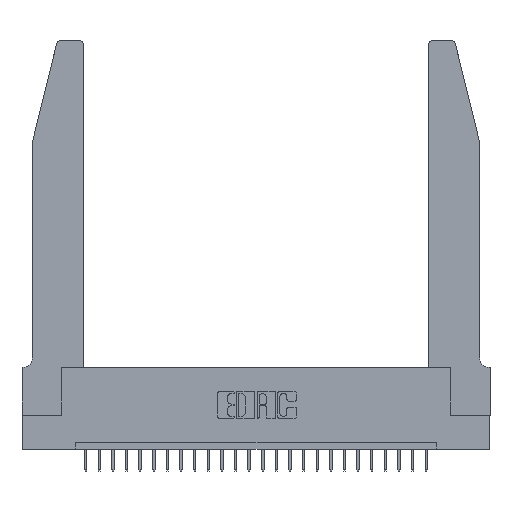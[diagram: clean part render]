
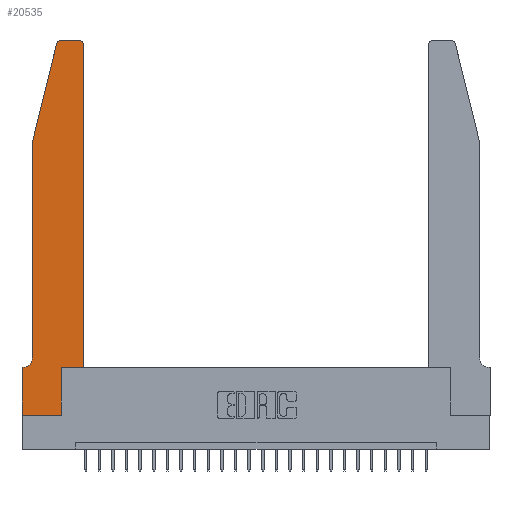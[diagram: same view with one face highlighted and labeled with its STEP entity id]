
A CAD part, top view. The second image highlights one B-rep face of the part: STEP entity #20535.
In plain terms, the highlighted planar face has unit normal (0, 0, 1).
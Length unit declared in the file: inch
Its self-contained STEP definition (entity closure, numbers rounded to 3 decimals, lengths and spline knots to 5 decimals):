
#472 = DIRECTION ( 'NONE',  ( -1., 0., 0. ) ) ;
#567 = CARTESIAN_POINT ( 'NONE',  ( 0.0055, 0.42, 0.37 ) ) ;
#782 = LINE ( 'NONE', #8113, #13665 ) ;
#947 = CARTESIAN_POINT ( 'NONE',  ( 0.25487, 2.72718, 0.37 ) ) ;
#1021 = EDGE_CURVE ( 'NONE', #4574, #17911, #22166, .T. ) ;
#1722 = DIRECTION ( 'NONE',  ( 1., 0., 0. ) ) ;
#2195 = CARTESIAN_POINT ( 'NONE',  ( 0.0055, 0.35, 0.37 ) ) ;
#2310 = AXIS2_PLACEMENT_3D ( 'NONE', #18141, #11943, #11862 ) ;
#2638 = CARTESIAN_POINT ( 'NONE',  ( 0.0755, 0.42, 0.37 ) ) ;
#2735 = DIRECTION ( 'NONE',  ( -1., 0., 0. ) ) ;
#2921 = ORIENTED_EDGE ( 'NONE', *, *, #15101, .T. ) ;
#3608 = ORIENTED_EDGE ( 'NONE', *, *, #18608, .T. ) ;
#3681 = EDGE_CURVE ( 'NONE', #5317, #7916, #22575, .T. ) ;
#3725 = DIRECTION ( 'NONE',  ( 0., 1., 0. ) ) ;
#4243 = AXIS2_PLACEMENT_3D ( 'NONE', #16172, #10070, #22353 ) ;
#4574 = VERTEX_POINT ( 'NONE', #26457 ) ;
#5047 = ORIENTED_EDGE ( 'NONE', *, *, #3681, .T. ) ;
#5179 = VECTOR ( 'NONE', #20657, 39.37008 ) ;
#5317 = VERTEX_POINT ( 'NONE', #20674 ) ;
#5391 = LINE ( 'NONE', #9657, #13701 ) ;
#5473 = DIRECTION ( 'NONE',  ( 1., 0., 0. ) ) ;
#5727 = CARTESIAN_POINT ( 'NONE',  ( 0., 0.35, 0.37 ) ) ;
#5961 = CARTESIAN_POINT ( 'NONE',  ( 0.4505, 0.35, 0.37 ) ) ;
#5993 = ORIENTED_EDGE ( 'NONE', *, *, #10647, .T. ) ;
#6028 = EDGE_LOOP ( 'NONE', ( #17126, #25659, #2921, #17463, #17440, #12930, #3608, #5993, #26164, #24307, #5047, #20089 ) ) ;
#6051 = DIRECTION ( 'NONE',  ( 0., 1., 0. ) ) ;
#6361 = CARTESIAN_POINT ( 'NONE',  ( 0.0755, 2., 0.37 ) ) ;
#6406 = CARTESIAN_POINT ( 'NONE',  ( 0., 0., 0.37 ) ) ;
#6776 = DIRECTION ( 'NONE',  ( 1., 0., 0. ) ) ;
#6785 = VERTEX_POINT ( 'NONE', #19899 ) ;
#7282 = CARTESIAN_POINT ( 'NONE',  ( 0., 0., 0.37 ) ) ;
#7431 = CARTESIAN_POINT ( 'NONE',  ( 0.0755, 2., 0.37 ) ) ;
#7916 = VERTEX_POINT ( 'NONE', #19694 ) ;
#8113 = CARTESIAN_POINT ( 'NONE',  ( 0.2865, 0.35, 0.37 ) ) ;
#8120 = VERTEX_POINT ( 'NONE', #23173 ) ;
#8487 = EDGE_CURVE ( 'NONE', #6785, #10697, #9330, .T. ) ;
#9235 = LINE ( 'NONE', #7431, #21674 ) ;
#9330 = LINE ( 'NONE', #6361, #5179 ) ;
#9657 = CARTESIAN_POINT ( 'NONE',  ( 0.0755, 0.35, 0.37 ) ) ;
#9749 = PLANE ( 'NONE',  #23344 ) ;
#10070 = DIRECTION ( 'NONE',  ( 0., 0., 1. ) ) ;
#10303 = CARTESIAN_POINT ( 'NONE',  ( 0., 0.35, 0.37 ) ) ;
#10463 = FACE_OUTER_BOUND ( 'NONE', #6028, .T. ) ;
#10647 = EDGE_CURVE ( 'NONE', #8120, #23838, #16918, .T. ) ;
#10697 = VERTEX_POINT ( 'NONE', #2638 ) ;
#11446 = VERTEX_POINT ( 'NONE', #10303 ) ;
#11862 = DIRECTION ( 'NONE',  ( 1., 0., 0. ) ) ;
#11943 = DIRECTION ( 'NONE',  ( 0., 0., 1. ) ) ;
#12259 = VERTEX_POINT ( 'NONE', #21391 ) ;
#12690 = EDGE_CURVE ( 'NONE', #20250, #4574, #12952, .T. ) ;
#12881 = EDGE_CURVE ( 'NONE', #10697, #16638, #26360, .T. ) ;
#12915 = CIRCLE ( 'NONE', #2310, 0.03 ) ;
#12930 = ORIENTED_EDGE ( 'NONE', *, *, #15286, .T. ) ;
#12952 = LINE ( 'NONE', #20877, #15826 ) ;
#13261 = CARTESIAN_POINT ( 'NONE',  ( 0.2865, 0., 0.37 ) ) ;
#13665 = VECTOR ( 'NONE', #3725, 39.37008 ) ;
#13701 = VECTOR ( 'NONE', #24636, 39.37008 ) ;
#15101 = EDGE_CURVE ( 'NONE', #17911, #6785, #9235, .T. ) ;
#15286 = EDGE_CURVE ( 'NONE', #16638, #11446, #5391, .T. ) ;
#15826 = VECTOR ( 'NONE', #472, 39.37008 ) ;
#16172 = CARTESIAN_POINT ( 'NONE',  ( 0.284, 2.72, 0.37 ) ) ;
#16638 = VERTEX_POINT ( 'NONE', #2195 ) ;
#16812 = DIRECTION ( 'NONE',  ( 0., 0., -1. ) ) ;
#16918 = LINE ( 'NONE', #6406, #26483 ) ;
#17126 = ORIENTED_EDGE ( 'NONE', *, *, #12690, .T. ) ;
#17440 = ORIENTED_EDGE ( 'NONE', *, *, #12881, .T. ) ;
#17463 = ORIENTED_EDGE ( 'NONE', *, *, #8487, .T. ) ;
#17612 = VECTOR ( 'NONE', #1722, 39.37008 ) ;
#17787 = DIRECTION ( 'NONE',  ( 0., -1., 0. ) ) ;
#17877 = VECTOR ( 'NONE', #6051, 39.37008 ) ;
#17911 = VERTEX_POINT ( 'NONE', #947 ) ;
#18014 = VECTOR ( 'NONE', #17787, 39.37008 ) ;
#18141 = CARTESIAN_POINT ( 'NONE',  ( 0.4205, 2.72, 0.37 ) ) ;
#18243 = CARTESIAN_POINT ( 'NONE',  ( 0.4505, 0.35, 0.37 ) ) ;
#18608 = EDGE_CURVE ( 'NONE', #11446, #8120, #24987, .T. ) ;
#18831 = AXIS2_PLACEMENT_3D ( 'NONE', #567, #16812, #2735 ) ;
#19694 = CARTESIAN_POINT ( 'NONE',  ( 0.4505, 2.72, 0.37 ) ) ;
#19899 = CARTESIAN_POINT ( 'NONE',  ( 0.0755, 2., 0.37 ) ) ;
#20089 = ORIENTED_EDGE ( 'NONE', *, *, #26072, .T. ) ;
#20250 = VERTEX_POINT ( 'NONE', #23260 ) ;
#20535 = ADVANCED_FACE ( 'NONE', ( #10463 ), #9749, .T. ) ;
#20618 = EDGE_CURVE ( 'NONE', #23838, #12259, #782, .T. ) ;
#20657 = DIRECTION ( 'NONE',  ( 0., -1., 0. ) ) ;
#20674 = CARTESIAN_POINT ( 'NONE',  ( 0.4505, 0.35, 0.37 ) ) ;
#20877 = CARTESIAN_POINT ( 'NONE',  ( 0.2605, 2.75, 0.37 ) ) ;
#21391 = CARTESIAN_POINT ( 'NONE',  ( 0.2865, 0.35, 0.37 ) ) ;
#21541 = DIRECTION ( 'NONE',  ( -0.239, -0.971, 0. ) ) ;
#21674 = VECTOR ( 'NONE', #21541, 39.37008 ) ;
#22030 = DIRECTION ( 'NONE',  ( 0., 0., 1. ) ) ;
#22166 = CIRCLE ( 'NONE', #4243, 0.03 ) ;
#22353 = DIRECTION ( 'NONE',  ( 1., 0., 0. ) ) ;
#22575 = LINE ( 'NONE', #5961, #17877 ) ;
#23027 = EDGE_CURVE ( 'NONE', #12259, #5317, #24512, .T. ) ;
#23173 = CARTESIAN_POINT ( 'NONE',  ( 0., 0., 0.37 ) ) ;
#23260 = CARTESIAN_POINT ( 'NONE',  ( 0.4205, 2.75, 0.37 ) ) ;
#23344 = AXIS2_PLACEMENT_3D ( 'NONE', #5727, #22030, #5473 ) ;
#23838 = VERTEX_POINT ( 'NONE', #13261 ) ;
#24307 = ORIENTED_EDGE ( 'NONE', *, *, #23027, .T. ) ;
#24512 = LINE ( 'NONE', #18243, #17612 ) ;
#24636 = DIRECTION ( 'NONE',  ( -1., 0., 0. ) ) ;
#24987 = LINE ( 'NONE', #7282, #18014 ) ;
#25659 = ORIENTED_EDGE ( 'NONE', *, *, #1021, .T. ) ;
#26072 = EDGE_CURVE ( 'NONE', #7916, #20250, #12915, .T. ) ;
#26164 = ORIENTED_EDGE ( 'NONE', *, *, #20618, .T. ) ;
#26360 = CIRCLE ( 'NONE', #18831, 0.07 ) ;
#26457 = CARTESIAN_POINT ( 'NONE',  ( 0.284, 2.75, 0.37 ) ) ;
#26483 = VECTOR ( 'NONE', #6776, 39.37008 ) ;
